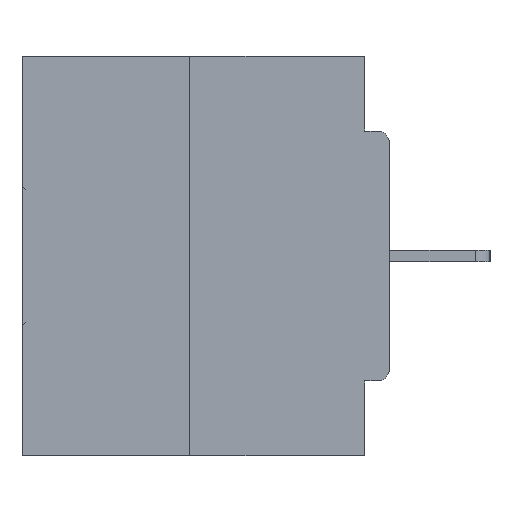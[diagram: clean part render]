
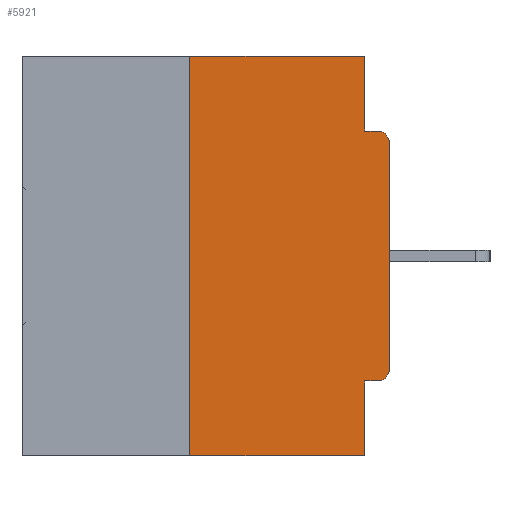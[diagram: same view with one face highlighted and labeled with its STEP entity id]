
A CAD part, left-side view. The second image highlights one B-rep face of the part: STEP entity #5921.
In plain terms, the highlighted planar face has unit normal (-1, 0, 0).
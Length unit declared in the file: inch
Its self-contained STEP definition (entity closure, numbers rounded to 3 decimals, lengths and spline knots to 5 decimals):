
#842 = EDGE_LOOP ( 'NONE', ( #17863, #17602, #3792, #33621, #29078, #27771, #26735, #9258, #18713, #11024 ) ) ;
#938 = DIRECTION ( 'NONE',  ( 0., 0., -1. ) ) ;
#1742 = EDGE_CURVE ( 'NONE', #17717, #36277, #3521, .T. ) ;
#2812 = AXIS2_PLACEMENT_3D ( 'NONE', #16240, #24323, #30227 ) ;
#2841 = EDGE_CURVE ( 'NONE', #29622, #26702, #28189, .T. ) ;
#2962 = CARTESIAN_POINT ( 'NONE',  ( 0., 0., 0. ) ) ;
#3309 = VECTOR ( 'NONE', #31620, 39.37008 ) ;
#3521 = LINE ( 'NONE', #17823, #25912 ) ;
#3628 = VERTEX_POINT ( 'NONE', #4575 ) ;
#3792 = ORIENTED_EDGE ( 'NONE', *, *, #2841, .T. ) ;
#4416 = DIRECTION ( 'NONE',  ( -1., 0., 0. ) ) ;
#4575 = CARTESIAN_POINT ( 'NONE',  ( 0., 0.015, -0.0935 ) ) ;
#5921 = ADVANCED_FACE ( 'NONE', ( #32978 ), #19185, .F. ) ;
#6165 = DIRECTION ( 'NONE',  ( 0., 0., 1. ) ) ;
#6491 = EDGE_CURVE ( 'NONE', #36327, #17975, #36068, .T. ) ;
#7437 = VECTOR ( 'NONE', #30904, 39.37008 ) ;
#8327 = VERTEX_POINT ( 'NONE', #29018 ) ;
#9094 = LINE ( 'NONE', #14406, #24386 ) ;
#9129 = EDGE_CURVE ( 'NONE', #27854, #36327, #18133, .T. ) ;
#9258 = ORIENTED_EDGE ( 'NONE', *, *, #35540, .T. ) ;
#10451 = DIRECTION ( 'NONE',  ( 0., 0., -1. ) ) ;
#11024 = ORIENTED_EDGE ( 'NONE', *, *, #1742, .F. ) ;
#11732 = EDGE_CURVE ( 'NONE', #30473, #17717, #31976, .T. ) ;
#12579 = EDGE_CURVE ( 'NONE', #8327, #26702, #9094, .T. ) ;
#12744 = LINE ( 'NONE', #35214, #26914 ) ;
#13604 = EDGE_CURVE ( 'NONE', #36277, #3628, #26039, .T. ) ;
#14148 = DIRECTION ( 'NONE',  ( 0., 0., -1. ) ) ;
#14406 = CARTESIAN_POINT ( 'NONE',  ( 0., 0.031, -0.5 ) ) ;
#14625 = CARTESIAN_POINT ( 'NONE',  ( 0., 0., -0.0935 ) ) ;
#15325 = CARTESIAN_POINT ( 'NONE',  ( 0., 0., -0.3915 ) ) ;
#16062 = CARTESIAN_POINT ( 'NONE',  ( 0., 0.031, -0.0935 ) ) ;
#16240 = CARTESIAN_POINT ( 'NONE',  ( 0., 0.46, 0. ) ) ;
#17602 = ORIENTED_EDGE ( 'NONE', *, *, #23196, .F. ) ;
#17717 = VERTEX_POINT ( 'NONE', #18369 ) ;
#17719 = LINE ( 'NONE', #20668, #21143 ) ;
#17823 = CARTESIAN_POINT ( 'NONE',  ( 0., 0.031, 0. ) ) ;
#17863 = ORIENTED_EDGE ( 'NONE', *, *, #11732, .F. ) ;
#17975 = VERTEX_POINT ( 'NONE', #28856 ) ;
#18133 = CIRCLE ( 'NONE', #34574, 0.015 ) ;
#18369 = CARTESIAN_POINT ( 'NONE',  ( 0., 0.031, 0. ) ) ;
#18713 = ORIENTED_EDGE ( 'NONE', *, *, #13604, .F. ) ;
#19185 = PLANE ( 'NONE',  #2812 ) ;
#20668 = CARTESIAN_POINT ( 'NONE',  ( 0., 0.25, 0. ) ) ;
#20775 = CARTESIAN_POINT ( 'NONE',  ( 0., 0.015, -0.3915 ) ) ;
#20930 = VECTOR ( 'NONE', #22569, 39.37008 ) ;
#21143 = VECTOR ( 'NONE', #6165, 39.37008 ) ;
#22569 = DIRECTION ( 'NONE',  ( 0., -1., 0. ) ) ;
#22892 = DIRECTION ( 'NONE',  ( 0., 0., -1. ) ) ;
#23196 = EDGE_CURVE ( 'NONE', #29622, #30473, #17719, .T. ) ;
#24323 = DIRECTION ( 'NONE',  ( 1., 0., 0. ) ) ;
#24386 = VECTOR ( 'NONE', #22892, 39.37008 ) ;
#25075 = CARTESIAN_POINT ( 'NONE',  ( 0., 0.25, 0. ) ) ;
#25912 = VECTOR ( 'NONE', #14148, 39.37008 ) ;
#26039 = LINE ( 'NONE', #14625, #20930 ) ;
#26567 = DIRECTION ( 'NONE',  ( 0., 1., 0. ) ) ;
#26646 = CARTESIAN_POINT ( 'NONE',  ( 0., 0.015, -0.4065 ) ) ;
#26702 = VERTEX_POINT ( 'NONE', #30303 ) ;
#26735 = ORIENTED_EDGE ( 'NONE', *, *, #6491, .T. ) ;
#26832 = AXIS2_PLACEMENT_3D ( 'NONE', #35844, #35666, #10451 ) ;
#26914 = VECTOR ( 'NONE', #26567, 39.37008 ) ;
#27638 = DIRECTION ( 'NONE',  ( 0., -1., 0. ) ) ;
#27771 = ORIENTED_EDGE ( 'NONE', *, *, #9129, .T. ) ;
#27854 = VERTEX_POINT ( 'NONE', #26646 ) ;
#27927 = CARTESIAN_POINT ( 'NONE',  ( 0., 0.25, -0.5 ) ) ;
#28189 = LINE ( 'NONE', #30396, #31086 ) ;
#28856 = CARTESIAN_POINT ( 'NONE',  ( 0., 0., -0.1085 ) ) ;
#29018 = CARTESIAN_POINT ( 'NONE',  ( 0., 0.031, -0.4065 ) ) ;
#29078 = ORIENTED_EDGE ( 'NONE', *, *, #36308, .F. ) ;
#29243 = CARTESIAN_POINT ( 'NONE',  ( 0., 0.46, 0. ) ) ;
#29622 = VERTEX_POINT ( 'NONE', #27927 ) ;
#30227 = DIRECTION ( 'NONE',  ( 0., 0., -1. ) ) ;
#30303 = CARTESIAN_POINT ( 'NONE',  ( 0., 0.031, -0.5 ) ) ;
#30396 = CARTESIAN_POINT ( 'NONE',  ( 0., 0.46, -0.5 ) ) ;
#30473 = VERTEX_POINT ( 'NONE', #25075 ) ;
#30904 = DIRECTION ( 'NONE',  ( 0., 0., 1. ) ) ;
#31086 = VECTOR ( 'NONE', #27638, 39.37008 ) ;
#31620 = DIRECTION ( 'NONE',  ( 0., -1., 0. ) ) ;
#31976 = LINE ( 'NONE', #29243, #3309 ) ;
#32978 = FACE_OUTER_BOUND ( 'NONE', #842, .T. ) ;
#33621 = ORIENTED_EDGE ( 'NONE', *, *, #12579, .F. ) ;
#34574 = AXIS2_PLACEMENT_3D ( 'NONE', #20775, #4416, #938 ) ;
#35214 = CARTESIAN_POINT ( 'NONE',  ( 0., 0., -0.4065 ) ) ;
#35540 = EDGE_CURVE ( 'NONE', #17975, #3628, #35651, .T. ) ;
#35651 = CIRCLE ( 'NONE', #26832, 0.015 ) ;
#35666 = DIRECTION ( 'NONE',  ( -1., 0., 0. ) ) ;
#35844 = CARTESIAN_POINT ( 'NONE',  ( 0., 0.015, -0.1085 ) ) ;
#36068 = LINE ( 'NONE', #2962, #7437 ) ;
#36277 = VERTEX_POINT ( 'NONE', #16062 ) ;
#36308 = EDGE_CURVE ( 'NONE', #27854, #8327, #12744, .T. ) ;
#36327 = VERTEX_POINT ( 'NONE', #15325 ) ;
